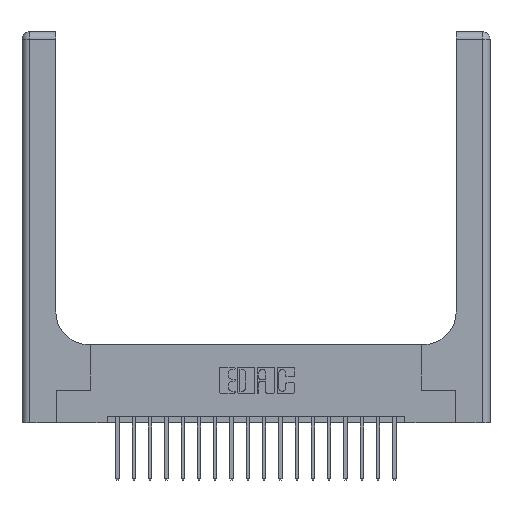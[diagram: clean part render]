
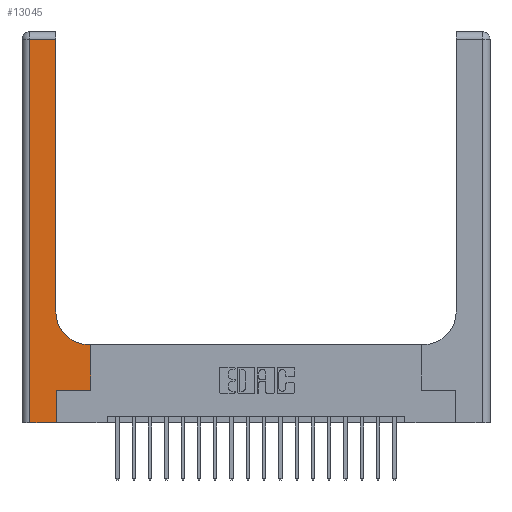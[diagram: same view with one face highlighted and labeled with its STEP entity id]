
A CAD part, top view. The second image highlights one B-rep face of the part: STEP entity #13045.
In plain terms, the highlighted planar face has unit normal (0, 0, 1).
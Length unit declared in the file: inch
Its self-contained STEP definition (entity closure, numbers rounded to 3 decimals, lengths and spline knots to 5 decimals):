
#15 = DIRECTION ( 'NONE',  ( 1., 0., 0. ) ) ;
#192 = CARTESIAN_POINT ( 'NONE',  ( 0.06, 2.94, 0.37 ) ) ;
#366 = EDGE_CURVE ( 'NONE', #13091, #9328, #16480, .T. ) ;
#478 = VERTEX_POINT ( 'NONE', #521 ) ;
#521 = CARTESIAN_POINT ( 'NONE',  ( 0.528, 0.25, 0.37 ) ) ;
#535 = CARTESIAN_POINT ( 'NONE',  ( 0., 2.94, 0.37 ) ) ;
#1127 = CARTESIAN_POINT ( 'NONE',  ( 0., 3., 0.37 ) ) ;
#1357 = CARTESIAN_POINT ( 'NONE',  ( 0.51, 0.85, 0.37 ) ) ;
#1674 = ORIENTED_EDGE ( 'NONE', *, *, #5125, .T. ) ;
#1882 = CARTESIAN_POINT ( 'NONE',  ( 0.26, 3., 0.37 ) ) ;
#1891 = VERTEX_POINT ( 'NONE', #3690 ) ;
#2100 = CARTESIAN_POINT ( 'NONE',  ( 0.51, 0.6, 0.37 ) ) ;
#2119 = CARTESIAN_POINT ( 'NONE',  ( 0.06, 0., 0.37 ) ) ;
#2315 = DIRECTION ( 'NONE',  ( -1., 0., 0. ) ) ;
#2359 = LINE ( 'NONE', #16832, #13226 ) ;
#2496 = ORIENTED_EDGE ( 'NONE', *, *, #6751, .T. ) ;
#2601 = VECTOR ( 'NONE', #2315, 39.37008 ) ;
#3090 = VERTEX_POINT ( 'NONE', #17558 ) ;
#3690 = CARTESIAN_POINT ( 'NONE',  ( 0.26, 2.94, 0.37 ) ) ;
#4145 = DIRECTION ( 'NONE',  ( 1., 0., 0. ) ) ;
#4555 = EDGE_CURVE ( 'NONE', #9328, #10918, #19954, .T. ) ;
#4779 = EDGE_LOOP ( 'NONE', ( #16044, #14154, #17606, #13039, #1674, #9797, #11191, #2496, #11935 ) ) ;
#4791 = CIRCLE ( 'NONE', #6761, 0.25 ) ;
#5125 = EDGE_CURVE ( 'NONE', #10918, #18495, #14794, .T. ) ;
#5578 = FACE_OUTER_BOUND ( 'NONE', #4779, .T. ) ;
#5700 = CARTESIAN_POINT ( 'NONE',  ( 0., 0., 0.37 ) ) ;
#6048 = EDGE_CURVE ( 'NONE', #478, #3090, #8692, .T. ) ;
#6311 = LINE ( 'NONE', #535, #2601 ) ;
#6418 = VERTEX_POINT ( 'NONE', #2100 ) ;
#6751 = EDGE_CURVE ( 'NONE', #3090, #6418, #2359, .T. ) ;
#6761 = AXIS2_PLACEMENT_3D ( 'NONE', #1357, #15542, #7733 ) ;
#6803 = DIRECTION ( 'NONE',  ( 0., -1., 0. ) ) ;
#7474 = VECTOR ( 'NONE', #11976, 39.37008 ) ;
#7506 = CARTESIAN_POINT ( 'NONE',  ( 0.265, 0., 0.37 ) ) ;
#7733 = DIRECTION ( 'NONE',  ( 1., 0., 0. ) ) ;
#7869 = EDGE_CURVE ( 'NONE', #1891, #13091, #6311, .T. ) ;
#8180 = CARTESIAN_POINT ( 'NONE',  ( 0.265, 0.25, 0.37 ) ) ;
#8692 = LINE ( 'NONE', #18243, #15819 ) ;
#9328 = VERTEX_POINT ( 'NONE', #2119 ) ;
#9797 = ORIENTED_EDGE ( 'NONE', *, *, #17494, .T. ) ;
#10918 = VERTEX_POINT ( 'NONE', #7506 ) ;
#11133 = VECTOR ( 'NONE', #6803, 39.37008 ) ;
#11191 = ORIENTED_EDGE ( 'NONE', *, *, #6048, .T. ) ;
#11675 = CARTESIAN_POINT ( 'NONE',  ( 0.265, 0., 0.37 ) ) ;
#11925 = PLANE ( 'NONE',  #15076 ) ;
#11935 = ORIENTED_EDGE ( 'NONE', *, *, #19160, .T. ) ;
#11976 = DIRECTION ( 'NONE',  ( 0., 1., 0. ) ) ;
#12304 = DIRECTION ( 'NONE',  ( -1., 0., 0. ) ) ;
#12706 = VECTOR ( 'NONE', #15, 39.37008 ) ;
#13039 = ORIENTED_EDGE ( 'NONE', *, *, #4555, .T. ) ;
#13045 = ADVANCED_FACE ( 'NONE', ( #5578 ), #11925, .F. ) ;
#13091 = VERTEX_POINT ( 'NONE', #192 ) ;
#13226 = VECTOR ( 'NONE', #13310, 39.37008 ) ;
#13255 = CARTESIAN_POINT ( 'NONE',  ( 0.06, 3., 0.37 ) ) ;
#13310 = DIRECTION ( 'NONE',  ( -1., 0., 0. ) ) ;
#13861 = DIRECTION ( 'NONE',  ( 0., 0., -1. ) ) ;
#14154 = ORIENTED_EDGE ( 'NONE', *, *, #7869, .T. ) ;
#14396 = LINE ( 'NONE', #1882, #14448 ) ;
#14448 = VECTOR ( 'NONE', #14500, 39.37008 ) ;
#14500 = DIRECTION ( 'NONE',  ( 0., 1., 0. ) ) ;
#14794 = LINE ( 'NONE', #11675, #7474 ) ;
#15043 = DIRECTION ( 'NONE',  ( 0., 1., 0. ) ) ;
#15076 = AXIS2_PLACEMENT_3D ( 'NONE', #1127, #13861, #12304 ) ;
#15542 = DIRECTION ( 'NONE',  ( 0., 0., -1. ) ) ;
#15819 = VECTOR ( 'NONE', #15043, 39.37008 ) ;
#15931 = CARTESIAN_POINT ( 'NONE',  ( 0.265, 0.25, 0.37 ) ) ;
#16044 = ORIENTED_EDGE ( 'NONE', *, *, #20359, .T. ) ;
#16480 = LINE ( 'NONE', #13255, #11133 ) ;
#16832 = CARTESIAN_POINT ( 'NONE',  ( 0.26, 0.6, 0.37 ) ) ;
#17088 = VERTEX_POINT ( 'NONE', #19122 ) ;
#17494 = EDGE_CURVE ( 'NONE', #18495, #478, #17527, .T. ) ;
#17527 = LINE ( 'NONE', #8180, #12706 ) ;
#17558 = CARTESIAN_POINT ( 'NONE',  ( 0.528, 0.6, 0.37 ) ) ;
#17606 = ORIENTED_EDGE ( 'NONE', *, *, #366, .T. ) ;
#18243 = CARTESIAN_POINT ( 'NONE',  ( 0.528, 0.25, 0.37 ) ) ;
#18382 = VECTOR ( 'NONE', #4145, 39.37008 ) ;
#18495 = VERTEX_POINT ( 'NONE', #15931 ) ;
#19122 = CARTESIAN_POINT ( 'NONE',  ( 0.26, 0.85, 0.37 ) ) ;
#19160 = EDGE_CURVE ( 'NONE', #6418, #17088, #4791, .T. ) ;
#19954 = LINE ( 'NONE', #5700, #18382 ) ;
#20359 = EDGE_CURVE ( 'NONE', #17088, #1891, #14396, .T. ) ;
